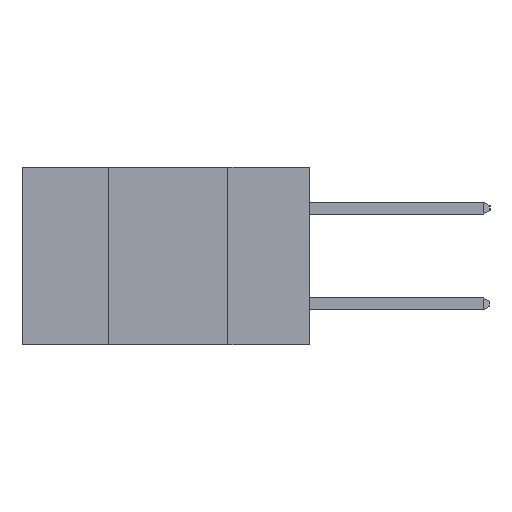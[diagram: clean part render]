
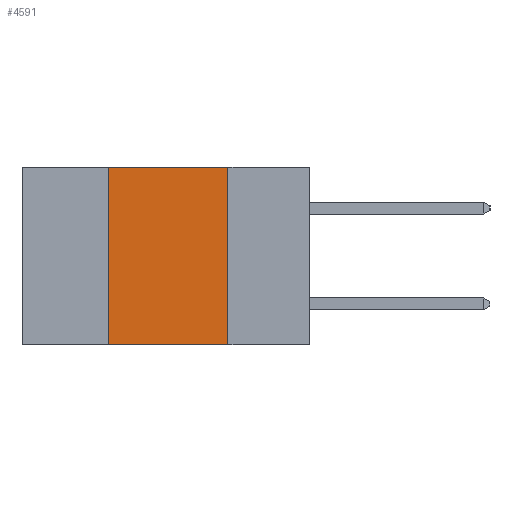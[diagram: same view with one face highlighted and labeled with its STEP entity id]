
A CAD part, left-side view. The second image highlights one B-rep face of the part: STEP entity #4591.
In plain terms, the highlighted planar face has unit normal (-1, 0, 0).
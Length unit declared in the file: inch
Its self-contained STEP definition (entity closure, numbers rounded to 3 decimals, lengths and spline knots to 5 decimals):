
#244 = VERTEX_POINT ( 'NONE', #1219 ) ;
#250 = LINE ( 'NONE', #307, #440 ) ;
#307 = CARTESIAN_POINT ( 'NONE',  ( 0., 0.42, 0. ) ) ;
#440 = VECTOR ( 'NONE', #3590, 39.37008 ) ;
#451 = ORIENTED_EDGE ( 'NONE', *, *, #4364, .F. ) ;
#467 = FACE_OUTER_BOUND ( 'NONE', #4034, .T. ) ;
#901 = VECTOR ( 'NONE', #3210, 39.37008 ) ;
#1015 = LINE ( 'NONE', #2711, #9855 ) ;
#1219 = CARTESIAN_POINT ( 'NONE',  ( 0., 0.17, 0. ) ) ;
#1444 = CARTESIAN_POINT ( 'NONE',  ( 0., 0.6, 0. ) ) ;
#1848 = CARTESIAN_POINT ( 'NONE',  ( 0., 0.42, 0. ) ) ;
#2301 = CARTESIAN_POINT ( 'NONE',  ( 0., 0.6, 0. ) ) ;
#2711 = CARTESIAN_POINT ( 'NONE',  ( 0., 0.6, -0.37 ) ) ;
#2943 = CARTESIAN_POINT ( 'NONE',  ( 0., 0.17, -0.37 ) ) ;
#3210 = DIRECTION ( 'NONE',  ( 0., -1., 0. ) ) ;
#3335 = ORIENTED_EDGE ( 'NONE', *, *, #7545, .F. ) ;
#3590 = DIRECTION ( 'NONE',  ( 0., 0., 1. ) ) ;
#3835 = VERTEX_POINT ( 'NONE', #10685 ) ;
#4034 = EDGE_LOOP ( 'NONE', ( #451, #7449, #3335, #9687 ) ) ;
#4103 = VERTEX_POINT ( 'NONE', #1848 ) ;
#4312 = DIRECTION ( 'NONE',  ( 0., 0., -1. ) ) ;
#4364 = EDGE_CURVE ( 'NONE', #244, #10282, #9756, .T. ) ;
#4369 = DIRECTION ( 'NONE',  ( 0., -1., 0. ) ) ;
#4382 = EDGE_CURVE ( 'NONE', #4103, #244, #8936, .T. ) ;
#4591 = ADVANCED_FACE ( 'NONE', ( #467 ), #4836, .F. ) ;
#4836 = PLANE ( 'NONE',  #10319 ) ;
#4858 = CARTESIAN_POINT ( 'NONE',  ( 0., 0.17, 0. ) ) ;
#7449 = ORIENTED_EDGE ( 'NONE', *, *, #4382, .F. ) ;
#7505 = EDGE_CURVE ( 'NONE', #3835, #10282, #1015, .T. ) ;
#7545 = EDGE_CURVE ( 'NONE', #3835, #4103, #250, .T. ) ;
#7823 = VECTOR ( 'NONE', #4312, 39.37008 ) ;
#8043 = DIRECTION ( 'NONE',  ( 1., 0., 0. ) ) ;
#8936 = LINE ( 'NONE', #1444, #901 ) ;
#9680 = DIRECTION ( 'NONE',  ( 0., 0., -1. ) ) ;
#9687 = ORIENTED_EDGE ( 'NONE', *, *, #7505, .T. ) ;
#9756 = LINE ( 'NONE', #4858, #7823 ) ;
#9855 = VECTOR ( 'NONE', #4369, 39.37008 ) ;
#10282 = VERTEX_POINT ( 'NONE', #2943 ) ;
#10319 = AXIS2_PLACEMENT_3D ( 'NONE', #2301, #8043, #9680 ) ;
#10685 = CARTESIAN_POINT ( 'NONE',  ( 0., 0.42, -0.37 ) ) ;
